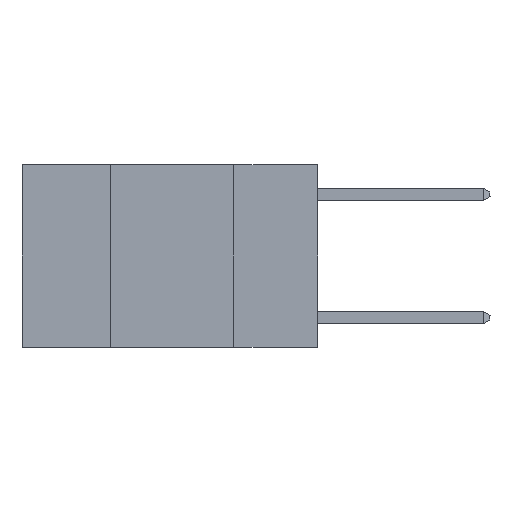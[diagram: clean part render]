
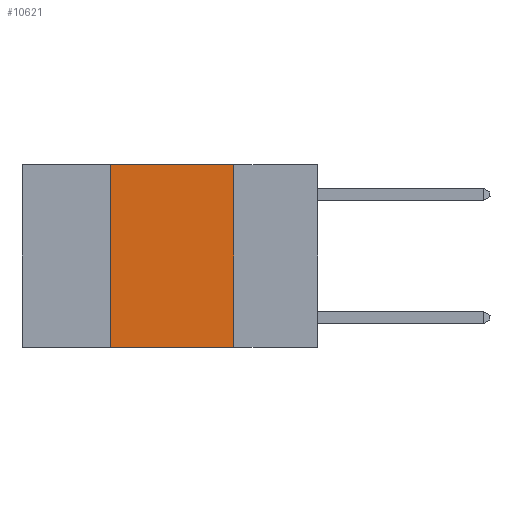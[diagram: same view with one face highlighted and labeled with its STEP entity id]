
A CAD part, left-side view. The second image highlights one B-rep face of the part: STEP entity #10621.
In plain terms, the highlighted planar face has unit normal (-1, 0, 0).
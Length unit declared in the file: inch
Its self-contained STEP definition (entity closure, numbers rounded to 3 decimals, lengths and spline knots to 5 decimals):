
#122 = EDGE_CURVE ( 'NONE', #5802, #20281, #2182, .T. ) ;
#550 = EDGE_LOOP ( 'NONE', ( #18449, #12539, #12650, #2114 ) ) ;
#1044 = VERTEX_POINT ( 'NONE', #5051 ) ;
#1736 = CARTESIAN_POINT ( 'NONE',  ( 0., 0.17, -0.37 ) ) ;
#1875 = FACE_OUTER_BOUND ( 'NONE', #550, .T. ) ;
#2114 = ORIENTED_EDGE ( 'NONE', *, *, #5384, .T. ) ;
#2182 = LINE ( 'NONE', #8278, #5449 ) ;
#3943 = VECTOR ( 'NONE', #6859, 39.37008 ) ;
#5051 = CARTESIAN_POINT ( 'NONE',  ( 0., 0.17, 0. ) ) ;
#5229 = CARTESIAN_POINT ( 'NONE',  ( 0., 0.17, 0. ) ) ;
#5384 = EDGE_CURVE ( 'NONE', #5802, #11749, #12236, .T. ) ;
#5435 = CARTESIAN_POINT ( 'NONE',  ( 0., 0.6, 0. ) ) ;
#5449 = VECTOR ( 'NONE', #12456, 39.37008 ) ;
#5802 = VERTEX_POINT ( 'NONE', #13122 ) ;
#5922 = CARTESIAN_POINT ( 'NONE',  ( 0., 0.6, 0. ) ) ;
#6196 = CARTESIAN_POINT ( 'NONE',  ( 0., 0.42, 0. ) ) ;
#6859 = DIRECTION ( 'NONE',  ( 0., 0., -1. ) ) ;
#7063 = DIRECTION ( 'NONE',  ( 0., 0., -1. ) ) ;
#7244 = AXIS2_PLACEMENT_3D ( 'NONE', #5435, #16438, #7063 ) ;
#8074 = EDGE_CURVE ( 'NONE', #20281, #1044, #12498, .T. ) ;
#8278 = CARTESIAN_POINT ( 'NONE',  ( 0., 0.42, 0. ) ) ;
#9043 = CARTESIAN_POINT ( 'NONE',  ( 0., 0.6, -0.37 ) ) ;
#10621 = ADVANCED_FACE ( 'NONE', ( #1875 ), #14815, .F. ) ;
#10639 = DIRECTION ( 'NONE',  ( 0., -1., 0. ) ) ;
#10749 = DIRECTION ( 'NONE',  ( 0., -1., 0. ) ) ;
#11749 = VERTEX_POINT ( 'NONE', #1736 ) ;
#12236 = LINE ( 'NONE', #9043, #12730 ) ;
#12456 = DIRECTION ( 'NONE',  ( 0., 0., 1. ) ) ;
#12498 = LINE ( 'NONE', #5922, #16095 ) ;
#12539 = ORIENTED_EDGE ( 'NONE', *, *, #8074, .F. ) ;
#12650 = ORIENTED_EDGE ( 'NONE', *, *, #122, .F. ) ;
#12730 = VECTOR ( 'NONE', #10639, 39.37008 ) ;
#12953 = LINE ( 'NONE', #5229, #3943 ) ;
#13122 = CARTESIAN_POINT ( 'NONE',  ( 0., 0.42, -0.37 ) ) ;
#13639 = EDGE_CURVE ( 'NONE', #1044, #11749, #12953, .T. ) ;
#14815 = PLANE ( 'NONE',  #7244 ) ;
#16095 = VECTOR ( 'NONE', #10749, 39.37008 ) ;
#16438 = DIRECTION ( 'NONE',  ( 1., 0., 0. ) ) ;
#18449 = ORIENTED_EDGE ( 'NONE', *, *, #13639, .F. ) ;
#20281 = VERTEX_POINT ( 'NONE', #6196 ) ;
